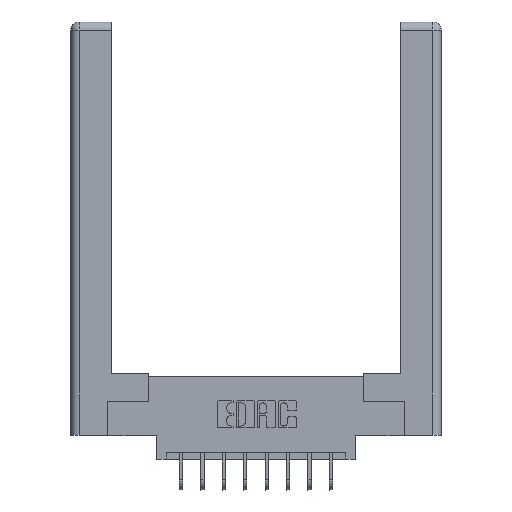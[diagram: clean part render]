
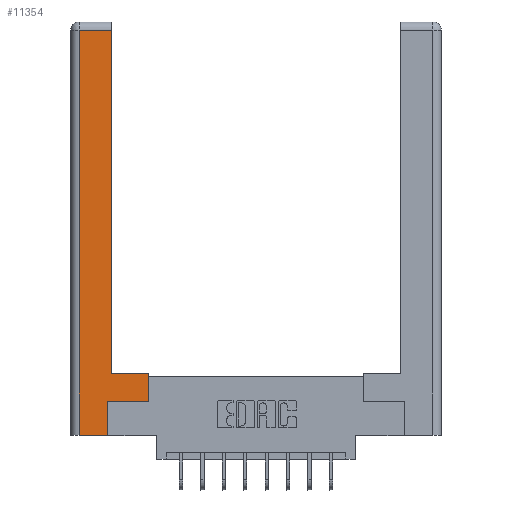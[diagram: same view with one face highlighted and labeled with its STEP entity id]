
A CAD part, top view. The second image highlights one B-rep face of the part: STEP entity #11354.
In plain terms, the highlighted planar face has unit normal (0, 0, 1).
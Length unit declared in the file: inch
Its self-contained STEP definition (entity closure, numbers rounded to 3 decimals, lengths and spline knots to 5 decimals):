
#297 = CARTESIAN_POINT ( 'NONE',  ( 0.265, 0.245, 0. ) ) ;
#485 = VERTEX_POINT ( 'NONE', #2829 ) ;
#526 = CARTESIAN_POINT ( 'NONE',  ( 0.0615, 0., 0. ) ) ;
#953 = VECTOR ( 'NONE', #1300, 39.37008 ) ;
#1059 = EDGE_CURVE ( 'NONE', #8776, #485, #7082, .T. ) ;
#1146 = ORIENTED_EDGE ( 'NONE', *, *, #8447, .T. ) ;
#1300 = DIRECTION ( 'NONE',  ( -1., 0., 0. ) ) ;
#1531 = ORIENTED_EDGE ( 'NONE', *, *, #8563, .T. ) ;
#1680 = PLANE ( 'NONE',  #10353 ) ;
#1714 = LINE ( 'NONE', #2289, #13044 ) ;
#1861 = CARTESIAN_POINT ( 'NONE',  ( 0.565, 0.45, 0. ) ) ;
#2289 = CARTESIAN_POINT ( 'NONE',  ( 0.0615, 0., 0. ) ) ;
#2555 = CARTESIAN_POINT ( 'NONE',  ( 0.295, 3., 0. ) ) ;
#2829 = CARTESIAN_POINT ( 'NONE',  ( 0.265, 0.245, 0. ) ) ;
#3194 = EDGE_CURVE ( 'NONE', #9333, #6660, #4069, .T. ) ;
#3295 = VECTOR ( 'NONE', #10980, 39.37008 ) ;
#3510 = CARTESIAN_POINT ( 'NONE',  ( 0.0615, 2.94, 0. ) ) ;
#3524 = ORIENTED_EDGE ( 'NONE', *, *, #3194, .T. ) ;
#3784 = DIRECTION ( 'NONE',  ( 0., 1., 0. ) ) ;
#3891 = DIRECTION ( 'NONE',  ( 0., 1., 0. ) ) ;
#3972 = VECTOR ( 'NONE', #14975, 39.37008 ) ;
#4044 = VECTOR ( 'NONE', #7441, 39.37008 ) ;
#4069 = LINE ( 'NONE', #14114, #953 ) ;
#4448 = CARTESIAN_POINT ( 'NONE',  ( 0.0615, 2.94, 0. ) ) ;
#4492 = ORIENTED_EDGE ( 'NONE', *, *, #11183, .T. ) ;
#4622 = EDGE_CURVE ( 'NONE', #6076, #9333, #6755, .T. ) ;
#5263 = ORIENTED_EDGE ( 'NONE', *, *, #4622, .T. ) ;
#5493 = FACE_OUTER_BOUND ( 'NONE', #5616, .T. ) ;
#5616 = EDGE_LOOP ( 'NONE', ( #1531, #1146, #4492, #12033, #14344, #10292, #5263, #3524 ) ) ;
#6076 = VERTEX_POINT ( 'NONE', #14846 ) ;
#6258 = VERTEX_POINT ( 'NONE', #4448 ) ;
#6660 = VERTEX_POINT ( 'NONE', #15039 ) ;
#6755 = LINE ( 'NONE', #8531, #4044 ) ;
#6910 = VECTOR ( 'NONE', #3784, 39.37008 ) ;
#7031 = DIRECTION ( 'NONE',  ( -1., 0., 0. ) ) ;
#7082 = LINE ( 'NONE', #297, #11480 ) ;
#7441 = DIRECTION ( 'NONE',  ( 0., 1., 0. ) ) ;
#7680 = VERTEX_POINT ( 'NONE', #12938 ) ;
#8447 = EDGE_CURVE ( 'NONE', #7680, #6258, #10237, .T. ) ;
#8531 = CARTESIAN_POINT ( 'NONE',  ( 0.565, 0.45, 0. ) ) ;
#8563 = EDGE_CURVE ( 'NONE', #6660, #7680, #10052, .T. ) ;
#8632 = CARTESIAN_POINT ( 'NONE',  ( 0.565, 0.245, 0. ) ) ;
#8775 = VECTOR ( 'NONE', #7031, 39.37008 ) ;
#8776 = VERTEX_POINT ( 'NONE', #11485 ) ;
#9267 = LINE ( 'NONE', #12604, #3972 ) ;
#9333 = VERTEX_POINT ( 'NONE', #1861 ) ;
#9441 = EDGE_CURVE ( 'NONE', #12543, #8776, #9267, .T. ) ;
#9887 = DIRECTION ( 'NONE',  ( 0., 0., -1. ) ) ;
#10052 = LINE ( 'NONE', #2555, #6910 ) ;
#10237 = LINE ( 'NONE', #3510, #8775 ) ;
#10292 = ORIENTED_EDGE ( 'NONE', *, *, #13169, .T. ) ;
#10353 = AXIS2_PLACEMENT_3D ( 'NONE', #10842, #9887, #14411 ) ;
#10842 = CARTESIAN_POINT ( 'NONE',  ( 0., 0., 0. ) ) ;
#10980 = DIRECTION ( 'NONE',  ( 1., 0., 0. ) ) ;
#11183 = EDGE_CURVE ( 'NONE', #6258, #12543, #1714, .T. ) ;
#11354 = ADVANCED_FACE ( 'NONE', ( #5493 ), #1680, .F. ) ;
#11480 = VECTOR ( 'NONE', #3891, 39.37008 ) ;
#11485 = CARTESIAN_POINT ( 'NONE',  ( 0.265, 0., 0. ) ) ;
#11498 = DIRECTION ( 'NONE',  ( 0., -1., 0. ) ) ;
#12033 = ORIENTED_EDGE ( 'NONE', *, *, #9441, .T. ) ;
#12543 = VERTEX_POINT ( 'NONE', #526 ) ;
#12604 = CARTESIAN_POINT ( 'NONE',  ( 0.265, 0., 0. ) ) ;
#12938 = CARTESIAN_POINT ( 'NONE',  ( 0.295, 2.94, 0. ) ) ;
#13044 = VECTOR ( 'NONE', #11498, 39.37008 ) ;
#13169 = EDGE_CURVE ( 'NONE', #485, #6076, #13418, .T. ) ;
#13418 = LINE ( 'NONE', #8632, #3295 ) ;
#14114 = CARTESIAN_POINT ( 'NONE',  ( 0.295, 0.45, 0. ) ) ;
#14344 = ORIENTED_EDGE ( 'NONE', *, *, #1059, .T. ) ;
#14411 = DIRECTION ( 'NONE',  ( -1., 0., 0. ) ) ;
#14846 = CARTESIAN_POINT ( 'NONE',  ( 0.565, 0.245, 0. ) ) ;
#14975 = DIRECTION ( 'NONE',  ( 1., 0., 0. ) ) ;
#15039 = CARTESIAN_POINT ( 'NONE',  ( 0.295, 0.45, 0. ) ) ;
